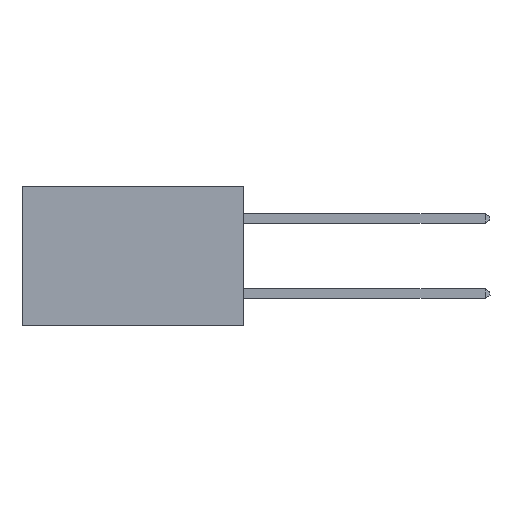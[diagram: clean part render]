
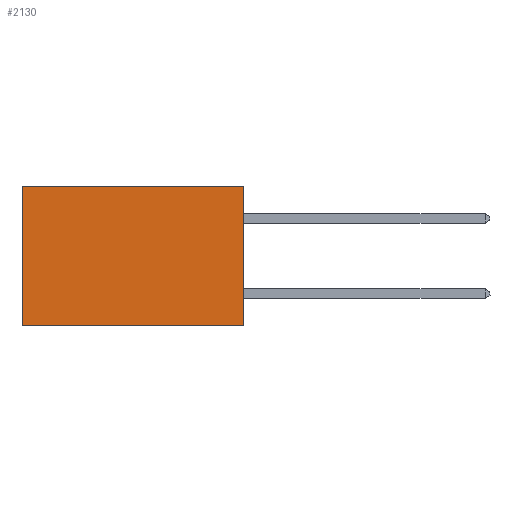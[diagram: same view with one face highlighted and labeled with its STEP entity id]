
A CAD part, left-side view. The second image highlights one B-rep face of the part: STEP entity #2130.
In plain terms, the highlighted planar face has unit normal (-1, 0, 0).
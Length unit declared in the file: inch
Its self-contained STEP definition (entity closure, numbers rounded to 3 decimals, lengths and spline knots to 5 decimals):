
#191 = VERTEX_POINT ( 'NONE', #608 ) ;
#218 = ORIENTED_EDGE ( 'NONE', *, *, #5823, .F. ) ;
#471 = CARTESIAN_POINT ( 'NONE',  ( 0.277, 0., 0. ) ) ;
#608 = CARTESIAN_POINT ( 'NONE',  ( 0.277, 0.59, 0. ) ) ;
#774 = EDGE_CURVE ( 'NONE', #6486, #191, #8308, .T. ) ;
#914 = DIRECTION ( 'NONE',  ( 0., 0., -1. ) ) ;
#1606 = VECTOR ( 'NONE', #13272, 39.37008 ) ;
#2130 = ADVANCED_FACE ( 'NONE', ( #10833 ), #5924, .F. ) ;
#2431 = DIRECTION ( 'NONE',  ( 0., 0., -1. ) ) ;
#2844 = ORIENTED_EDGE ( 'NONE', *, *, #10502, .F. ) ;
#3075 = EDGE_LOOP ( 'NONE', ( #3395, #218, #2844, #7670 ) ) ;
#3327 = LINE ( 'NONE', #8620, #11813 ) ;
#3395 = ORIENTED_EDGE ( 'NONE', *, *, #10593, .T. ) ;
#3445 = DIRECTION ( 'NONE',  ( 1., 0., 0. ) ) ;
#4614 = CARTESIAN_POINT ( 'NONE',  ( 0.277, 0.59, -0.37 ) ) ;
#4621 = CARTESIAN_POINT ( 'NONE',  ( 0.277, 0., -0.37 ) ) ;
#5823 = EDGE_CURVE ( 'NONE', #9410, #11622, #11311, .T. ) ;
#5924 = PLANE ( 'NONE',  #10253 ) ;
#5976 = CARTESIAN_POINT ( 'NONE',  ( 0.277, 0., -0.37 ) ) ;
#6486 = VERTEX_POINT ( 'NONE', #471 ) ;
#6690 = CARTESIAN_POINT ( 'NONE',  ( 0.277, 0., 0. ) ) ;
#7212 = CARTESIAN_POINT ( 'NONE',  ( 0.277, 0., -0.37 ) ) ;
#7374 = DIRECTION ( 'NONE',  ( 0., 1., 0. ) ) ;
#7513 = DIRECTION ( 'NONE',  ( 0., 0., -1. ) ) ;
#7670 = ORIENTED_EDGE ( 'NONE', *, *, #774, .T. ) ;
#8256 = LINE ( 'NONE', #14160, #10805 ) ;
#8308 = LINE ( 'NONE', #6690, #1606 ) ;
#8620 = CARTESIAN_POINT ( 'NONE',  ( 0.277, 0., -0.37 ) ) ;
#8753 = VECTOR ( 'NONE', #7374, 39.37008 ) ;
#9410 = VERTEX_POINT ( 'NONE', #4621 ) ;
#10253 = AXIS2_PLACEMENT_3D ( 'NONE', #5976, #3445, #2431 ) ;
#10502 = EDGE_CURVE ( 'NONE', #6486, #9410, #3327, .T. ) ;
#10593 = EDGE_CURVE ( 'NONE', #191, #11622, #8256, .T. ) ;
#10805 = VECTOR ( 'NONE', #914, 39.37008 ) ;
#10833 = FACE_OUTER_BOUND ( 'NONE', #3075, .T. ) ;
#11311 = LINE ( 'NONE', #7212, #8753 ) ;
#11622 = VERTEX_POINT ( 'NONE', #4614 ) ;
#11813 = VECTOR ( 'NONE', #7513, 39.37008 ) ;
#13272 = DIRECTION ( 'NONE',  ( 0., 1., 0. ) ) ;
#14160 = CARTESIAN_POINT ( 'NONE',  ( 0.277, 0.59, -0.37 ) ) ;
